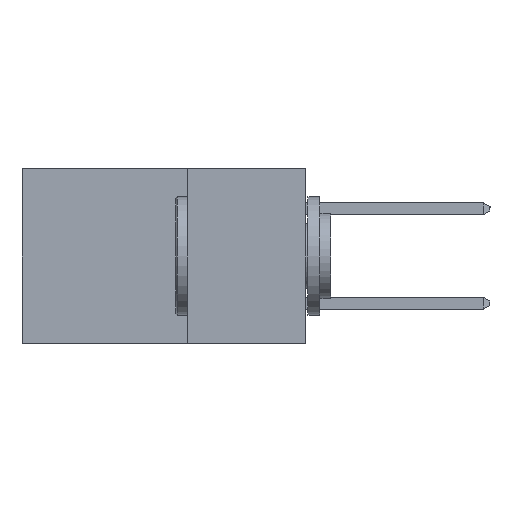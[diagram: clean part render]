
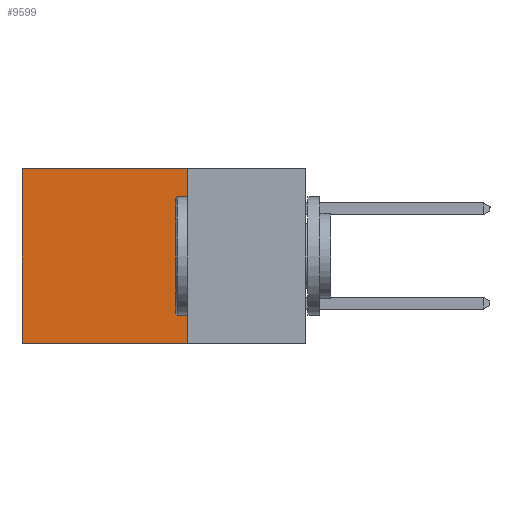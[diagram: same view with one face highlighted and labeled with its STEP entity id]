
A CAD part, left-side view. The second image highlights one B-rep face of the part: STEP entity #9599.
In plain terms, the highlighted planar face has unit normal (-1, 0, 0).
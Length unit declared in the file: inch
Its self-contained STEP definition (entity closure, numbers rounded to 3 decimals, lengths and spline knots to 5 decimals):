
#1094 = ORIENTED_EDGE ( 'NONE', *, *, #13980, .T. ) ;
#2402 = LINE ( 'NONE', #14537, #11701 ) ;
#2612 = AXIS2_PLACEMENT_3D ( 'NONE', #20795, #5649, #7858 ) ;
#2915 = ORIENTED_EDGE ( 'NONE', *, *, #7808, .T. ) ;
#3307 = EDGE_LOOP ( 'NONE', ( #2915, #20159, #5363, #1094 ) ) ;
#3342 = DIRECTION ( 'NONE',  ( 0., 1., 0. ) ) ;
#3555 = DIRECTION ( 'NONE',  ( 0., 0., -1. ) ) ;
#3977 = CARTESIAN_POINT ( 'NONE',  ( 0.2615, 0.6, 0. ) ) ;
#5363 = ORIENTED_EDGE ( 'NONE', *, *, #21627, .F. ) ;
#5501 = FACE_OUTER_BOUND ( 'NONE', #3307, .T. ) ;
#5649 = DIRECTION ( 'NONE',  ( 1., 0., 0. ) ) ;
#7063 = CARTESIAN_POINT ( 'NONE',  ( 0.2615, 0.25, 0. ) ) ;
#7300 = VECTOR ( 'NONE', #3555, 39.37008 ) ;
#7380 = VECTOR ( 'NONE', #13986, 39.37008 ) ;
#7808 = EDGE_CURVE ( 'NONE', #8071, #21495, #18006, .T. ) ;
#7858 = DIRECTION ( 'NONE',  ( 0., 0., -1. ) ) ;
#8071 = VERTEX_POINT ( 'NONE', #3977 ) ;
#8882 = VERTEX_POINT ( 'NONE', #9971 ) ;
#9297 = CARTESIAN_POINT ( 'NONE',  ( 0.2615, 0.6, -0.37 ) ) ;
#9599 = ADVANCED_FACE ( 'NONE', ( #5501 ), #12409, .F. ) ;
#9971 = CARTESIAN_POINT ( 'NONE',  ( 0.2615, 0.25, -0.37 ) ) ;
#11701 = VECTOR ( 'NONE', #22950, 39.37008 ) ;
#11925 = LINE ( 'NONE', #16454, #7380 ) ;
#12409 = PLANE ( 'NONE',  #2612 ) ;
#13980 = EDGE_CURVE ( 'NONE', #20534, #8071, #2402, .T. ) ;
#13986 = DIRECTION ( 'NONE',  ( 0., 0., -1. ) ) ;
#14537 = CARTESIAN_POINT ( 'NONE',  ( 0.2615, 0.25, 0. ) ) ;
#15804 = CARTESIAN_POINT ( 'NONE',  ( 0.2615, 0.6, -0.37 ) ) ;
#16454 = CARTESIAN_POINT ( 'NONE',  ( 0.2615, 0.25, -0.37 ) ) ;
#18006 = LINE ( 'NONE', #15804, #7300 ) ;
#18064 = LINE ( 'NONE', #24830, #25155 ) ;
#20159 = ORIENTED_EDGE ( 'NONE', *, *, #26196, .F. ) ;
#20534 = VERTEX_POINT ( 'NONE', #7063 ) ;
#20795 = CARTESIAN_POINT ( 'NONE',  ( 0.2615, 0.25, -0.37 ) ) ;
#21495 = VERTEX_POINT ( 'NONE', #9297 ) ;
#21627 = EDGE_CURVE ( 'NONE', #20534, #8882, #11925, .T. ) ;
#22950 = DIRECTION ( 'NONE',  ( 0., 1., 0. ) ) ;
#24830 = CARTESIAN_POINT ( 'NONE',  ( 0.2615, 0.25, -0.37 ) ) ;
#25155 = VECTOR ( 'NONE', #3342, 39.37008 ) ;
#26196 = EDGE_CURVE ( 'NONE', #8882, #21495, #18064, .T. ) ;
